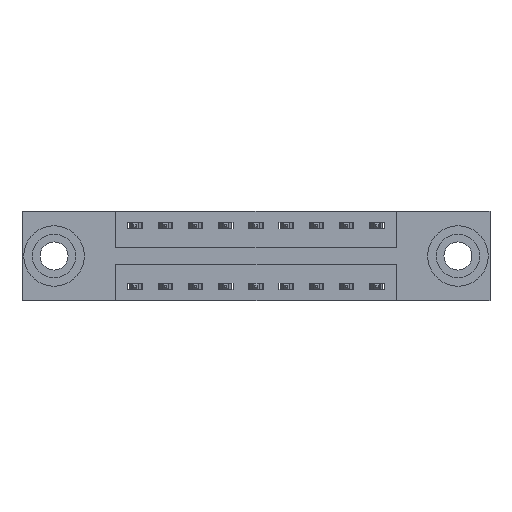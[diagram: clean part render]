
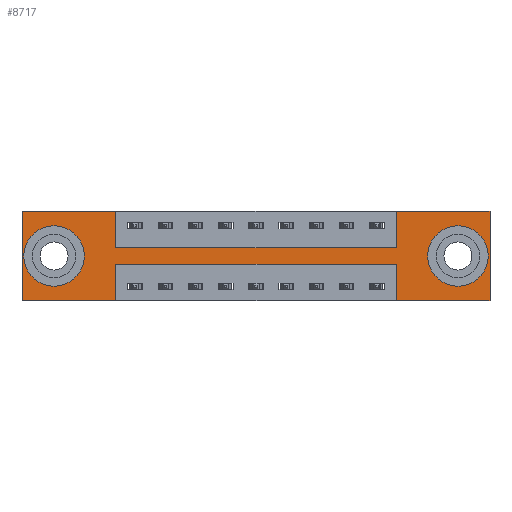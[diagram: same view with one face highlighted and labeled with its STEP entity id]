
A CAD part, front view. The second image highlights one B-rep face of the part: STEP entity #8717.
In plain terms, the highlighted planar face has unit normal (0, -1, 0).
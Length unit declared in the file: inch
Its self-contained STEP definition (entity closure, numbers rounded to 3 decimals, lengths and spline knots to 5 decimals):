
#25 = VERTEX_POINT ( 'NONE', #9364 ) ;
#113 = ORIENTED_EDGE ( 'NONE', *, *, #3499, .T. ) ;
#393 = ORIENTED_EDGE ( 'NONE', *, *, #6009, .F. ) ;
#426 = ORIENTED_EDGE ( 'NONE', *, *, #5354, .F. ) ;
#466 = LINE ( 'NONE', #9762, #2653 ) ;
#834 = ORIENTED_EDGE ( 'NONE', *, *, #2120, .F. ) ;
#838 = VECTOR ( 'NONE', #10884, 39.37008 ) ;
#882 = VERTEX_POINT ( 'NONE', #1511 ) ;
#1096 = CARTESIAN_POINT ( 'NONE',  ( 1.5475, 0., -0.15 ) ) ;
#1133 = ORIENTED_EDGE ( 'NONE', *, *, #6479, .F. ) ;
#1164 = DIRECTION ( 'NONE',  ( -1., 0., 0. ) ) ;
#1436 = LINE ( 'NONE', #5113, #8004 ) ;
#1501 = ORIENTED_EDGE ( 'NONE', *, *, #5564, .T. ) ;
#1506 = DIRECTION ( 'NONE',  ( 0., 1., 0. ) ) ;
#1511 = CARTESIAN_POINT ( 'NONE',  ( 1.8025, 0., -0.263 ) ) ;
#1626 = FACE_OUTER_BOUND ( 'NONE', #4226, .T. ) ;
#1653 = ORIENTED_EDGE ( 'NONE', *, *, #4714, .F. ) ;
#1710 = CARTESIAN_POINT ( 'NONE',  ( 0.1325, 0., -0.185 ) ) ;
#1725 = VECTOR ( 'NONE', #9145, 39.37008 ) ;
#1802 = DIRECTION ( 'NONE',  ( 0., -1., 0. ) ) ;
#2050 = ORIENTED_EDGE ( 'NONE', *, *, #4638, .F. ) ;
#2120 = EDGE_CURVE ( 'NONE', #8147, #4592, #466, .T. ) ;
#2193 = VERTEX_POINT ( 'NONE', #7231 ) ;
#2228 = LINE ( 'NONE', #4730, #10845 ) ;
#2293 = LINE ( 'NONE', #6729, #10911 ) ;
#2419 = CARTESIAN_POINT ( 'NONE',  ( 0.1325, 0., -0.107 ) ) ;
#2420 = LINE ( 'NONE', #5178, #3803 ) ;
#2444 = CARTESIAN_POINT ( 'NONE',  ( 1.8025, 0., -0.185 ) ) ;
#2457 = DIRECTION ( 'NONE',  ( -1., 0., 0. ) ) ;
#2538 = CARTESIAN_POINT ( 'NONE',  ( 0., 0., 0. ) ) ;
#2624 = DIRECTION ( 'NONE',  ( 0., 0., 1. ) ) ;
#2653 = VECTOR ( 'NONE', #9619, 39.37008 ) ;
#2683 = CARTESIAN_POINT ( 'NONE',  ( 1.5475, 0., -0.37 ) ) ;
#2925 = CIRCLE ( 'NONE', #6817, 0.078 ) ;
#3265 = LINE ( 'NONE', #2538, #838 ) ;
#3345 = DIRECTION ( 'NONE',  ( 0., 0., -1. ) ) ;
#3351 = ORIENTED_EDGE ( 'NONE', *, *, #7475, .T. ) ;
#3499 = EDGE_CURVE ( 'NONE', #882, #10398, #10453, .T. ) ;
#3515 = DIRECTION ( 'NONE',  ( 0., 1., 0. ) ) ;
#3560 = CARTESIAN_POINT ( 'NONE',  ( 1.5475, 0., -0.22 ) ) ;
#3587 = PLANE ( 'NONE',  #9454 ) ;
#3753 = ORIENTED_EDGE ( 'NONE', *, *, #6731, .F. ) ;
#3803 = VECTOR ( 'NONE', #6014, 39.37008 ) ;
#3836 = AXIS2_PLACEMENT_3D ( 'NONE', #2444, #8361, #3345 ) ;
#4078 = VERTEX_POINT ( 'NONE', #8548 ) ;
#4169 = CARTESIAN_POINT ( 'NONE',  ( 0.3875, 0., 0. ) ) ;
#4226 = EDGE_LOOP ( 'NONE', ( #1133, #6529, #5717, #5448, #4308, #1653, #834, #7405, #3753, #393, #426, #2050 ) ) ;
#4308 = ORIENTED_EDGE ( 'NONE', *, *, #5464, .F. ) ;
#4486 = EDGE_CURVE ( 'NONE', #5899, #8147, #2293, .T. ) ;
#4490 = CARTESIAN_POINT ( 'NONE',  ( 0., 0., -0.37 ) ) ;
#4497 = VERTEX_POINT ( 'NONE', #2419 ) ;
#4524 = VECTOR ( 'NONE', #7418, 39.37008 ) ;
#4533 = CIRCLE ( 'NONE', #8145, 0.078 ) ;
#4592 = VERTEX_POINT ( 'NONE', #10810 ) ;
#4596 = LINE ( 'NONE', #8777, #8974 ) ;
#4638 = EDGE_CURVE ( 'NONE', #6212, #4078, #1436, .T. ) ;
#4649 = EDGE_LOOP ( 'NONE', ( #3351, #9595 ) ) ;
#4714 = EDGE_CURVE ( 'NONE', #4592, #7938, #3265, .T. ) ;
#4730 = CARTESIAN_POINT ( 'NONE',  ( 0.3875, 0., -0.37 ) ) ;
#4747 = VERTEX_POINT ( 'NONE', #9294 ) ;
#4996 = CARTESIAN_POINT ( 'NONE',  ( 1.935, 0., -0.37 ) ) ;
#5046 = LINE ( 'NONE', #5141, #9144 ) ;
#5113 = CARTESIAN_POINT ( 'NONE',  ( 0., 0., -0.37 ) ) ;
#5141 = CARTESIAN_POINT ( 'NONE',  ( 1.935, 0., 0. ) ) ;
#5178 = CARTESIAN_POINT ( 'NONE',  ( 0., 0., -0.37 ) ) ;
#5337 = AXIS2_PLACEMENT_3D ( 'NONE', #1710, #7716, #2624 ) ;
#5354 = EDGE_CURVE ( 'NONE', #4078, #2193, #10662, .T. ) ;
#5363 = VERTEX_POINT ( 'NONE', #4996 ) ;
#5364 = CARTESIAN_POINT ( 'NONE',  ( 1.935, 0., 0. ) ) ;
#5448 = ORIENTED_EDGE ( 'NONE', *, *, #5510, .F. ) ;
#5464 = EDGE_CURVE ( 'NONE', #7938, #5363, #5046, .T. ) ;
#5510 = EDGE_CURVE ( 'NONE', #5363, #8697, #2420, .T. ) ;
#5542 = CARTESIAN_POINT ( 'NONE',  ( 1.8025, 0., -0.107 ) ) ;
#5554 = DIRECTION ( 'NONE',  ( 0., 0., -1. ) ) ;
#5564 = EDGE_CURVE ( 'NONE', #10398, #882, #4533, .T. ) ;
#5717 = ORIENTED_EDGE ( 'NONE', *, *, #6325, .F. ) ;
#5793 = LINE ( 'NONE', #2683, #6071 ) ;
#5894 = CARTESIAN_POINT ( 'NONE',  ( 0., 0., 0. ) ) ;
#5899 = VERTEX_POINT ( 'NONE', #6381 ) ;
#5970 = DIRECTION ( 'NONE',  ( 0., 0., -1. ) ) ;
#6009 = EDGE_CURVE ( 'NONE', #2193, #25, #8894, .T. ) ;
#6014 = DIRECTION ( 'NONE',  ( -1., 0., 0. ) ) ;
#6061 = CARTESIAN_POINT ( 'NONE',  ( 0.3875, 0., -0.22 ) ) ;
#6071 = VECTOR ( 'NONE', #8515, 39.37008 ) ;
#6212 = VERTEX_POINT ( 'NONE', #6858 ) ;
#6325 = EDGE_CURVE ( 'NONE', #8697, #10164, #5793, .T. ) ;
#6381 = CARTESIAN_POINT ( 'NONE',  ( 0.3875, 0., -0.15 ) ) ;
#6479 = EDGE_CURVE ( 'NONE', #6931, #6212, #2228, .T. ) ;
#6481 = EDGE_CURVE ( 'NONE', #10164, #6931, #4596, .T. ) ;
#6529 = ORIENTED_EDGE ( 'NONE', *, *, #6481, .F. ) ;
#6590 = CARTESIAN_POINT ( 'NONE',  ( 0., 0., 0. ) ) ;
#6690 = DIRECTION ( 'NONE',  ( 0., 0., -1. ) ) ;
#6721 = CARTESIAN_POINT ( 'NONE',  ( 0.1325, 0., -0.185 ) ) ;
#6729 = CARTESIAN_POINT ( 'NONE',  ( 0.3875, 0., -0.15 ) ) ;
#6731 = EDGE_CURVE ( 'NONE', #25, #5899, #8552, .T. ) ;
#6817 = AXIS2_PLACEMENT_3D ( 'NONE', #6721, #1506, #7532 ) ;
#6858 = CARTESIAN_POINT ( 'NONE',  ( 0.3875, 0., -0.37 ) ) ;
#6910 = EDGE_CURVE ( 'NONE', #4747, #4497, #8684, .T. ) ;
#6931 = VERTEX_POINT ( 'NONE', #6061 ) ;
#7231 = CARTESIAN_POINT ( 'NONE',  ( 0., 0., 0. ) ) ;
#7405 = ORIENTED_EDGE ( 'NONE', *, *, #4486, .F. ) ;
#7418 = DIRECTION ( 'NONE',  ( 1., 0., 0. ) ) ;
#7475 = EDGE_CURVE ( 'NONE', #4497, #4747, #2925, .T. ) ;
#7532 = DIRECTION ( 'NONE',  ( 0., 0., 1. ) ) ;
#7716 = DIRECTION ( 'NONE',  ( 0., 1., 0. ) ) ;
#7799 = DIRECTION ( 'NONE',  ( 0., 0., -1. ) ) ;
#7938 = VERTEX_POINT ( 'NONE', #5364 ) ;
#8004 = VECTOR ( 'NONE', #2457, 39.37008 ) ;
#8145 = AXIS2_PLACEMENT_3D ( 'NONE', #8495, #3515, #9320 ) ;
#8147 = VERTEX_POINT ( 'NONE', #1096 ) ;
#8361 = DIRECTION ( 'NONE',  ( 0., 1., 0. ) ) ;
#8419 = FACE_BOUND ( 'NONE', #10408, .T. ) ;
#8495 = CARTESIAN_POINT ( 'NONE',  ( 1.8025, 0., -0.185 ) ) ;
#8515 = DIRECTION ( 'NONE',  ( 0., 0., 1. ) ) ;
#8548 = CARTESIAN_POINT ( 'NONE',  ( 0., 0., -0.37 ) ) ;
#8552 = LINE ( 'NONE', #4169, #8825 ) ;
#8672 = FACE_BOUND ( 'NONE', #4649, .T. ) ;
#8684 = CIRCLE ( 'NONE', #5337, 0.078 ) ;
#8697 = VERTEX_POINT ( 'NONE', #9350 ) ;
#8717 = ADVANCED_FACE ( 'NONE', ( #8419, #8672, #1626 ), #3587, .T. ) ;
#8777 = CARTESIAN_POINT ( 'NONE',  ( 0.3875, 0., -0.22 ) ) ;
#8825 = VECTOR ( 'NONE', #6690, 39.37008 ) ;
#8894 = LINE ( 'NONE', #6590, #4524 ) ;
#8974 = VECTOR ( 'NONE', #1164, 39.37008 ) ;
#9144 = VECTOR ( 'NONE', #5970, 39.37008 ) ;
#9145 = DIRECTION ( 'NONE',  ( 0., 0., 1. ) ) ;
#9294 = CARTESIAN_POINT ( 'NONE',  ( 0.1325, 0., -0.263 ) ) ;
#9320 = DIRECTION ( 'NONE',  ( 0., 0., -1. ) ) ;
#9350 = CARTESIAN_POINT ( 'NONE',  ( 1.5475, 0., -0.37 ) ) ;
#9364 = CARTESIAN_POINT ( 'NONE',  ( 0.3875, 0., 0. ) ) ;
#9454 = AXIS2_PLACEMENT_3D ( 'NONE', #4490, #1802, #7799 ) ;
#9595 = ORIENTED_EDGE ( 'NONE', *, *, #6910, .T. ) ;
#9619 = DIRECTION ( 'NONE',  ( 0., 0., 1. ) ) ;
#9762 = CARTESIAN_POINT ( 'NONE',  ( 1.5475, 0., 0. ) ) ;
#10164 = VERTEX_POINT ( 'NONE', #3560 ) ;
#10398 = VERTEX_POINT ( 'NONE', #5542 ) ;
#10408 = EDGE_LOOP ( 'NONE', ( #1501, #113 ) ) ;
#10453 = CIRCLE ( 'NONE', #3836, 0.078 ) ;
#10662 = LINE ( 'NONE', #5894, #1725 ) ;
#10743 = DIRECTION ( 'NONE',  ( 1., 0., 0. ) ) ;
#10810 = CARTESIAN_POINT ( 'NONE',  ( 1.5475, 0., 0. ) ) ;
#10845 = VECTOR ( 'NONE', #5554, 39.37008 ) ;
#10884 = DIRECTION ( 'NONE',  ( 1., 0., 0. ) ) ;
#10911 = VECTOR ( 'NONE', #10743, 39.37008 ) ;
